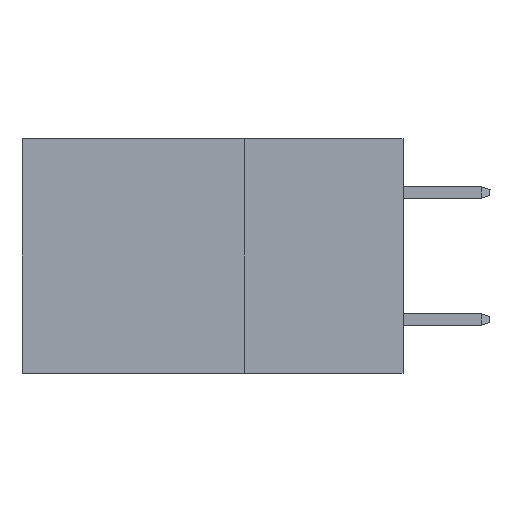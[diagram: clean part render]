
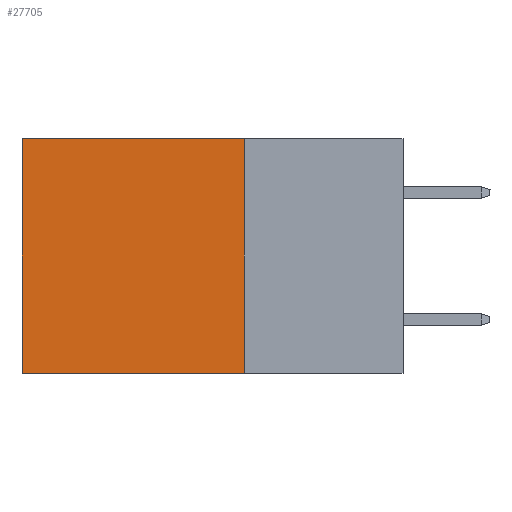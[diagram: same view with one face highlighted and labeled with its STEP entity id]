
A CAD part, left-side view. The second image highlights one B-rep face of the part: STEP entity #27705.
In plain terms, the highlighted planar face has unit normal (-1, 0, 0).
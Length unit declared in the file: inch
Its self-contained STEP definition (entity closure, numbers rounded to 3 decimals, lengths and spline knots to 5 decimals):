
#299 = VERTEX_POINT ( 'NONE', #39570 ) ;
#801 = PLANE ( 'NONE',  #28660 ) ;
#4763 = LINE ( 'NONE', #12346, #22601 ) ;
#7331 = CARTESIAN_POINT ( 'NONE',  ( 0.2875, 0.6, 0. ) ) ;
#8904 = CARTESIAN_POINT ( 'NONE',  ( 0.2875, 0.25, -0.37 ) ) ;
#9077 = VECTOR ( 'NONE', #41823, 39.37008 ) ;
#9640 = FACE_OUTER_BOUND ( 'NONE', #36146, .T. ) ;
#10131 = VERTEX_POINT ( 'NONE', #33028 ) ;
#10487 = DIRECTION ( 'NONE',  ( 0., 0., -1. ) ) ;
#11112 = CARTESIAN_POINT ( 'NONE',  ( 0.2875, 0.6, 0. ) ) ;
#11166 = CARTESIAN_POINT ( 'NONE',  ( 0.2875, 0.25, 0. ) ) ;
#11625 = VECTOR ( 'NONE', #23359, 39.37008 ) ;
#12346 = CARTESIAN_POINT ( 'NONE',  ( 0.2875, 0.25, 0. ) ) ;
#12349 = VERTEX_POINT ( 'NONE', #11112 ) ;
#14374 = DIRECTION ( 'NONE',  ( 1., 0., 0. ) ) ;
#14905 = ORIENTED_EDGE ( 'NONE', *, *, #38814, .T. ) ;
#16096 = ORIENTED_EDGE ( 'NONE', *, *, #19566, .F. ) ;
#16485 = VECTOR ( 'NONE', #40631, 39.37008 ) ;
#16609 = ORIENTED_EDGE ( 'NONE', *, *, #29335, .F. ) ;
#17057 = ORIENTED_EDGE ( 'NONE', *, *, #19790, .T. ) ;
#17121 = CARTESIAN_POINT ( 'NONE',  ( 0.2875, 0.25, 0. ) ) ;
#19566 = EDGE_CURVE ( 'NONE', #31637, #10131, #4763, .T. ) ;
#19790 = EDGE_CURVE ( 'NONE', #31637, #12349, #27738, .T. ) ;
#21567 = LINE ( 'NONE', #7331, #9077 ) ;
#22601 = VECTOR ( 'NONE', #40617, 39.37008 ) ;
#23359 = DIRECTION ( 'NONE',  ( 0., 1., 0. ) ) ;
#27705 = ADVANCED_FACE ( 'NONE', ( #9640 ), #801, .F. ) ;
#27738 = LINE ( 'NONE', #17121, #11625 ) ;
#28660 = AXIS2_PLACEMENT_3D ( 'NONE', #11166, #14374, #10487 ) ;
#29335 = EDGE_CURVE ( 'NONE', #10131, #299, #33950, .T. ) ;
#31637 = VERTEX_POINT ( 'NONE', #37267 ) ;
#33028 = CARTESIAN_POINT ( 'NONE',  ( 0.2875, 0.25, -0.37 ) ) ;
#33950 = LINE ( 'NONE', #8904, #16485 ) ;
#36146 = EDGE_LOOP ( 'NONE', ( #14905, #16609, #16096, #17057 ) ) ;
#37267 = CARTESIAN_POINT ( 'NONE',  ( 0.2875, 0.25, 0. ) ) ;
#38814 = EDGE_CURVE ( 'NONE', #12349, #299, #21567, .T. ) ;
#39570 = CARTESIAN_POINT ( 'NONE',  ( 0.2875, 0.6, -0.37 ) ) ;
#40617 = DIRECTION ( 'NONE',  ( 0., 0., -1. ) ) ;
#40631 = DIRECTION ( 'NONE',  ( 0., 1., 0. ) ) ;
#41823 = DIRECTION ( 'NONE',  ( 0., 0., -1. ) ) ;
